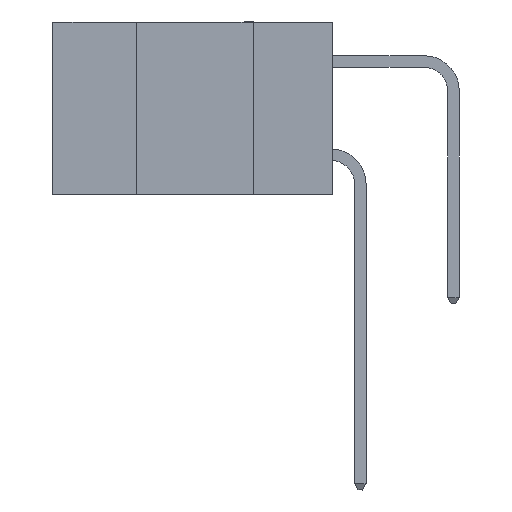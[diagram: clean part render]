
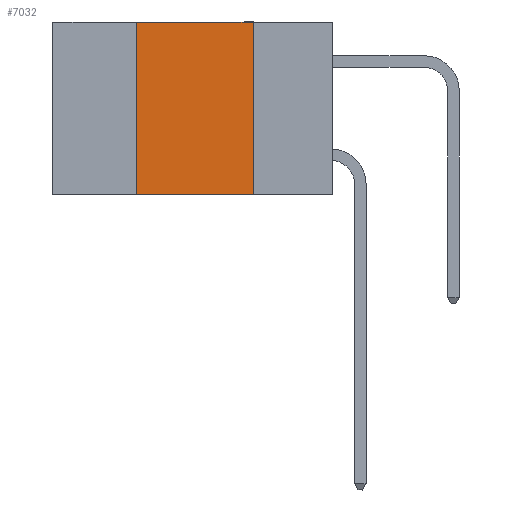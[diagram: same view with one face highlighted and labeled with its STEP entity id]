
A CAD part, left-side view. The second image highlights one B-rep face of the part: STEP entity #7032.
In plain terms, the highlighted planar face has unit normal (-1, 0, 0).
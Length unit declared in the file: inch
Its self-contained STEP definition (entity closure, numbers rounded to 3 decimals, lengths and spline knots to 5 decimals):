
#907 = EDGE_CURVE ( 'NONE', #11095, #2212, #17603, .T. ) ;
#977 = ORIENTED_EDGE ( 'NONE', *, *, #22417, .F. ) ;
#2118 = ORIENTED_EDGE ( 'NONE', *, *, #13656, .F. ) ;
#2212 = VERTEX_POINT ( 'NONE', #2581 ) ;
#2581 = CARTESIAN_POINT ( 'NONE',  ( 0., 0.17, -0.37 ) ) ;
#3226 = VECTOR ( 'NONE', #18313, 39.37008 ) ;
#3379 = LINE ( 'NONE', #24326, #4602 ) ;
#4408 = VERTEX_POINT ( 'NONE', #16788 ) ;
#4423 = CARTESIAN_POINT ( 'NONE',  ( 0., 0.6, -0.37 ) ) ;
#4466 = DIRECTION ( 'NONE',  ( 1., 0., 0. ) ) ;
#4602 = VECTOR ( 'NONE', #6879, 39.37008 ) ;
#6879 = DIRECTION ( 'NONE',  ( 0., 0., 1. ) ) ;
#7032 = ADVANCED_FACE ( 'NONE', ( #17765 ), #22117, .F. ) ;
#7869 = LINE ( 'NONE', #8560, #8777 ) ;
#8371 = DIRECTION ( 'NONE',  ( 0., -1., 0. ) ) ;
#8560 = CARTESIAN_POINT ( 'NONE',  ( 0., 0.17, 0. ) ) ;
#8777 = VECTOR ( 'NONE', #12605, 39.37008 ) ;
#10179 = ORIENTED_EDGE ( 'NONE', *, *, #13180, .F. ) ;
#10300 = CARTESIAN_POINT ( 'NONE',  ( 0., 0.6, 0. ) ) ;
#10471 = CARTESIAN_POINT ( 'NONE',  ( 0., 0.42, -0.37 ) ) ;
#11095 = VERTEX_POINT ( 'NONE', #10471 ) ;
#12441 = VECTOR ( 'NONE', #8371, 39.37008 ) ;
#12605 = DIRECTION ( 'NONE',  ( 0., 0., -1. ) ) ;
#12754 = ORIENTED_EDGE ( 'NONE', *, *, #907, .T. ) ;
#13180 = EDGE_CURVE ( 'NONE', #4408, #2212, #7869, .T. ) ;
#13656 = EDGE_CURVE ( 'NONE', #17469, #4408, #13659, .T. ) ;
#13659 = LINE ( 'NONE', #21654, #3226 ) ;
#16788 = CARTESIAN_POINT ( 'NONE',  ( 0., 0.17, 0. ) ) ;
#16940 = CARTESIAN_POINT ( 'NONE',  ( 0., 0.42, 0. ) ) ;
#17469 = VERTEX_POINT ( 'NONE', #16940 ) ;
#17603 = LINE ( 'NONE', #4423, #12441 ) ;
#17765 = FACE_OUTER_BOUND ( 'NONE', #20967, .T. ) ;
#18313 = DIRECTION ( 'NONE',  ( 0., -1., 0. ) ) ;
#18789 = AXIS2_PLACEMENT_3D ( 'NONE', #10300, #4466, #20131 ) ;
#20131 = DIRECTION ( 'NONE',  ( 0., 0., -1. ) ) ;
#20967 = EDGE_LOOP ( 'NONE', ( #10179, #2118, #977, #12754 ) ) ;
#21654 = CARTESIAN_POINT ( 'NONE',  ( 0., 0.6, 0. ) ) ;
#22117 = PLANE ( 'NONE',  #18789 ) ;
#22417 = EDGE_CURVE ( 'NONE', #11095, #17469, #3379, .T. ) ;
#24326 = CARTESIAN_POINT ( 'NONE',  ( 0., 0.42, 0. ) ) ;
